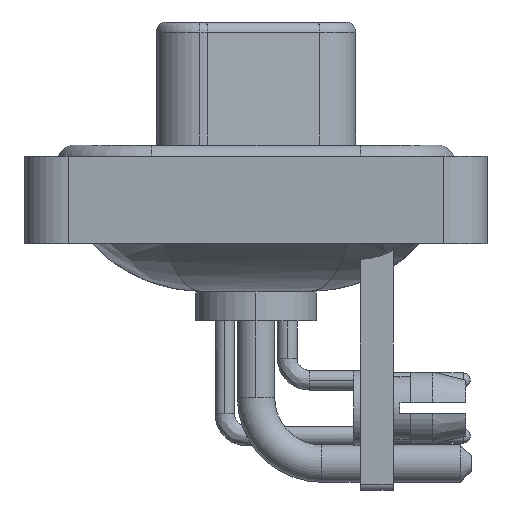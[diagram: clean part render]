
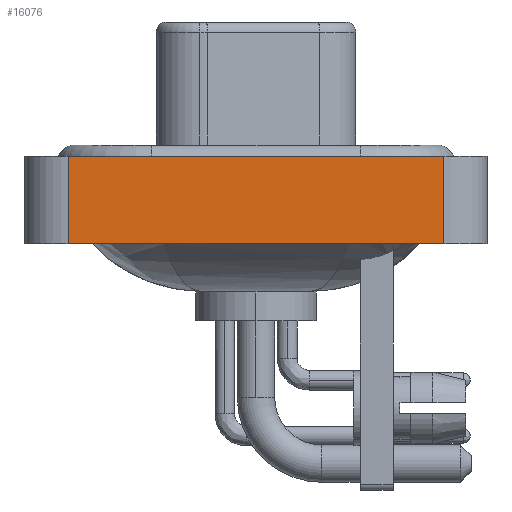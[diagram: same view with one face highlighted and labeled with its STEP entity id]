
A CAD part, left-side view. The second image highlights one B-rep face of the part: STEP entity #16076.
In plain terms, the highlighted planar face has unit normal (-1, 0, 0).
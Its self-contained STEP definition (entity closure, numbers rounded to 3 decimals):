
#131 = EDGE_LOOP ( 'NONE', ( #13665, #27725, #2086, #23853 ) ) ;
#488 = EDGE_CURVE ( 'NONE', #25123, #21472, #22860, .T. ) ;
#1223 = VERTEX_POINT ( 'NONE', #9071 ) ;
#2086 = ORIENTED_EDGE ( 'NONE', *, *, #488, .F. ) ;
#3008 = FACE_OUTER_BOUND ( 'NONE', #131, .T. ) ;
#3707 = DIRECTION ( 'NONE',  ( 0., 0., 1. ) ) ;
#3873 = CARTESIAN_POINT ( 'NONE',  ( -7.35, 8.55, -3.6 ) ) ;
#4291 = VERTEX_POINT ( 'NONE', #20262 ) ;
#4635 = CARTESIAN_POINT ( 'NONE',  ( -7.35, 8.55, -3.6 ) ) ;
#6777 = LINE ( 'NONE', #25787, #11068 ) ;
#7977 = DIRECTION ( 'NONE',  ( 0., 0., 1. ) ) ;
#9071 = CARTESIAN_POINT ( 'NONE',  ( -7.35, -8.55, 0.4 ) ) ;
#10650 = VECTOR ( 'NONE', #26192, 1000. ) ;
#11068 = VECTOR ( 'NONE', #19052, 1000. ) ;
#11430 = EDGE_CURVE ( 'NONE', #21472, #1223, #6777, .T. ) ;
#12938 = LINE ( 'NONE', #27719, #29385 ) ;
#13173 = VECTOR ( 'NONE', #3707, 1000. ) ;
#13665 = ORIENTED_EDGE ( 'NONE', *, *, #15251, .T. ) ;
#14534 = DIRECTION ( 'NONE',  ( -1., 0., 0. ) ) ;
#15251 = EDGE_CURVE ( 'NONE', #4291, #1223, #24005, .T. ) ;
#16076 = ADVANCED_FACE ( 'NONE', ( #3008 ), #29026, .T. ) ;
#18097 = AXIS2_PLACEMENT_3D ( 'NONE', #28733, #14534, #7977 ) ;
#19052 = DIRECTION ( 'NONE',  ( 0., -1., 0. ) ) ;
#20262 = CARTESIAN_POINT ( 'NONE',  ( -7.35, -8.55, -3.6 ) ) ;
#21267 = CARTESIAN_POINT ( 'NONE',  ( -7.35, 8.55, 0.4 ) ) ;
#21472 = VERTEX_POINT ( 'NONE', #21267 ) ;
#21663 = CARTESIAN_POINT ( 'NONE',  ( -7.35, -8.55, -3.6 ) ) ;
#22860 = LINE ( 'NONE', #3873, #13173 ) ;
#23853 = ORIENTED_EDGE ( 'NONE', *, *, #29224, .T. ) ;
#24005 = LINE ( 'NONE', #21663, #10650 ) ;
#25123 = VERTEX_POINT ( 'NONE', #4635 ) ;
#25787 = CARTESIAN_POINT ( 'NONE',  ( -7.35, -8.55, 0.4 ) ) ;
#26192 = DIRECTION ( 'NONE',  ( 0., 0., 1. ) ) ;
#27719 = CARTESIAN_POINT ( 'NONE',  ( -7.35, -8.55, -3.6 ) ) ;
#27725 = ORIENTED_EDGE ( 'NONE', *, *, #11430, .F. ) ;
#28733 = CARTESIAN_POINT ( 'NONE',  ( -7.35, -8.55, -3.6 ) ) ;
#29026 = PLANE ( 'NONE',  #18097 ) ;
#29224 = EDGE_CURVE ( 'NONE', #25123, #4291, #12938, .T. ) ;
#29385 = VECTOR ( 'NONE', #29759, 1000. ) ;
#29759 = DIRECTION ( 'NONE',  ( 0., -1., 0. ) ) ;
